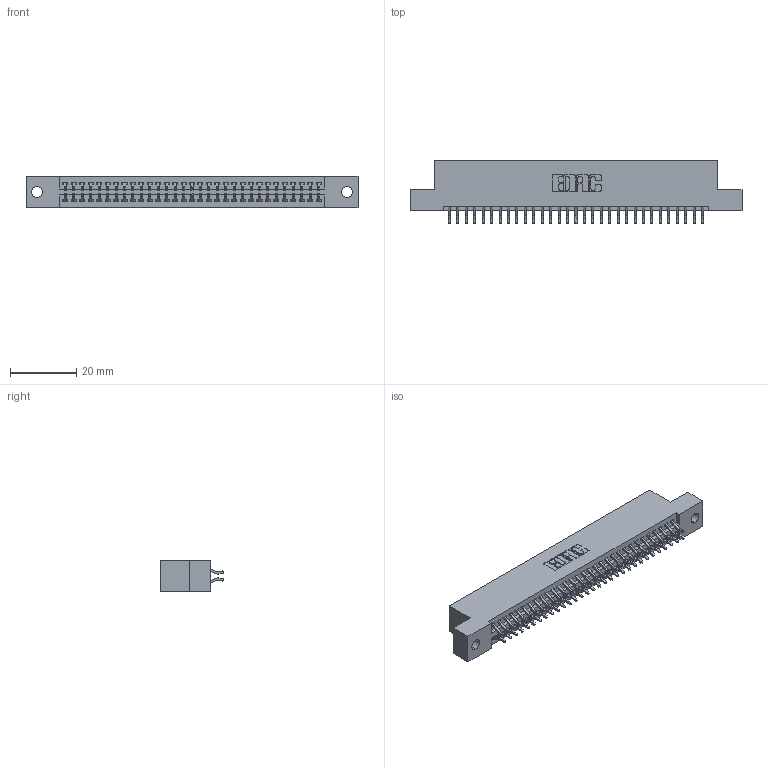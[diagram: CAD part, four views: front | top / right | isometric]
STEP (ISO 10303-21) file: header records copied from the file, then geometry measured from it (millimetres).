
FILE_DESCRIPTION (( 'STEP AP203' ), '1' );
FILE_NAME ('345-062-556-202.STEP', '2019-10-30T12:09:02', ( '' ), ( '' ), 'SwSTEP 2.0', 'SolidWorks 2016', '' );
FILE_SCHEMA (( 'CONFIG_CONTROL_DESIGN' ));
Length unit declared in the file: inch
Products named in the file (3): 345 Part_Flush Mounting Lugs - 0.128 Dia; 345-062-556-202; 345-292-001_556 Tail
Assembly tree (63 placements, depth 2):
  345-062-556-202
    345 Part_Flush Mounting Lugs - 0.128 Dia
    345-292-001_556 Tail  x62
Bounding box: 99.95 x 19.24 x 9.4 mm (x, y, z)
Volume: 9567.9 mm3; surface area: 13602.9 mm2
Topology: 63 solids, 63 shells, 3598 faces, 10695 edges, 7046 vertices
Faces by surface type: plane 2374, cylinder 1224
Entity records: 26027 total; most frequent: CARTESIAN_POINT 4388, ORIENTED_EDGE 4310, DIRECTION 3871, EDGE_CURVE 2155, LINE 1891, VECTOR 1891, VERTEX_POINT 1434, AXIS2_PLACEMENT_3D 990
